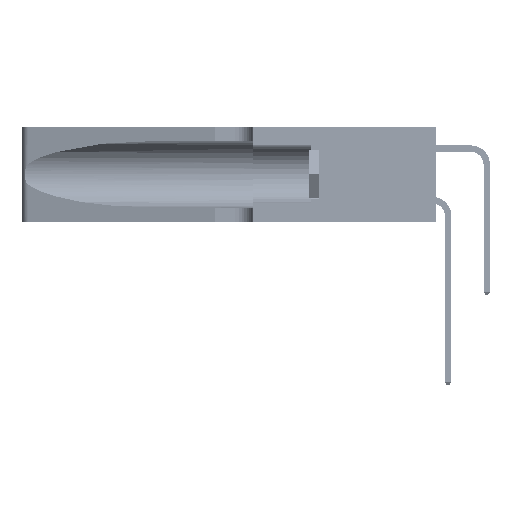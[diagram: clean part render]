
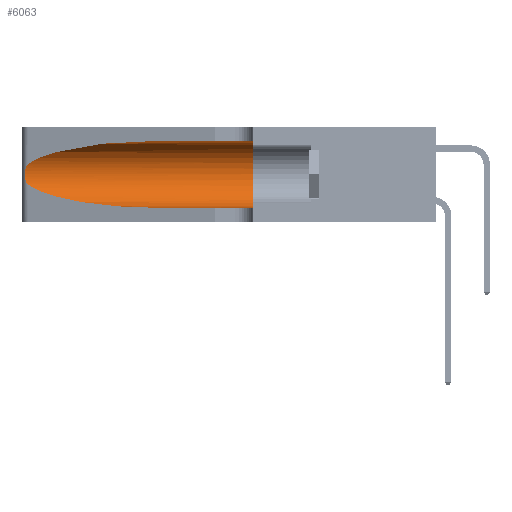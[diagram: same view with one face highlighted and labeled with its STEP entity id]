
A CAD part, left-side view. The second image highlights one B-rep face of the part: STEP entity #6063.
In plain terms, the highlighted cylindrical face has radius 3.308 mm (diameter 6.617 mm), a partial arc.
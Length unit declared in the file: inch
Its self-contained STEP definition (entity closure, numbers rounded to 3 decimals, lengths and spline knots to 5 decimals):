
#1471 = ORIENTED_EDGE ( 'NONE', *, *, #25149, .F. ) ;
#2690 = FACE_OUTER_BOUND ( 'NONE', #3818, .T. ) ;
#2762 = VERTEX_POINT ( 'NONE', #18186 ) ;
#2952 = CARTESIAN_POINT ( 'NONE',  ( 0.1305, 0.72297, 0.31525 ) ) ;
#3171 = CARTESIAN_POINT ( 'NONE',  ( 0.25787, 1.23484, 0.2124 ) ) ;
#3818 = EDGE_LOOP ( 'NONE', ( #35676, #42272, #21327, #41845, #1471, #45018 ) ) ;
#6063 = ADVANCED_FACE ( 'NONE', ( #2690 ), #40799, .F. ) ;
#6064 = AXIS2_PLACEMENT_3D ( 'NONE', #36379, #12071, #40425 ) ;
#6579 = EDGE_CURVE ( 'NONE', #7386, #30615, #22213, .T. ) ;
#7031 = DIRECTION ( 'NONE',  ( 0., 0., -1. ) ) ;
#7288 = CARTESIAN_POINT ( 'NONE',  ( 0.26018, 1.23835, 0.19895 ) ) ;
#7386 = VERTEX_POINT ( 'NONE', #46970 ) ;
#10471 =( BOUNDED_CURVE ( )  B_SPLINE_CURVE ( 3, ( #13249, #37545, #45640, #21408 ),
 .UNSPECIFIED., .F., .F. ) 
 B_SPLINE_CURVE_WITH_KNOTS ( ( 4, 4 ),
 ( 1.5708, 2.84003 ),
 .UNSPECIFIED. ) 
 CURVE ( )  GEOMETRIC_REPRESENTATION_ITEM ( )  RATIONAL_B_SPLINE_CURVE ( ( 1., 0.87, 0.87, 1. ) ) 
 REPRESENTATION_ITEM ( '' )  );
#11381 = CARTESIAN_POINT ( 'NONE',  ( 0.26075, 1.23896, 0.178 ) ) ;
#12071 = DIRECTION ( 'NONE',  ( 0., 1., 0. ) ) ;
#13249 = CARTESIAN_POINT ( 'NONE',  ( 0.1305, 0.72297, 0.31525 ) ) ;
#15060 = DIRECTION ( 'NONE',  ( 0., -1., 0. ) ) ;
#15468 = CARTESIAN_POINT ( 'NONE',  ( 0.25856, 1.23593, 0.16098 ) ) ;
#16273 = CARTESIAN_POINT ( 'NONE',  ( 0.25487, 1.22718, 0.22369 ) ) ;
#18186 = CARTESIAN_POINT ( 'NONE',  ( 0.1305, 0.35, 0.31525 ) ) ;
#18216 = CARTESIAN_POINT ( 'NONE',  ( 0.18966, 0.96281, 0.05475 ) ) ;
#18312 = B_SPLINE_CURVE_WITH_KNOTS ( 'NONE', 3,
 ( #43625, #39561, #27516, #3171, #31611, #7288, #35682, #11381, #39742, #15468, #43801, #19581, #47858, #23642 ),
 .UNSPECIFIED., .F., .F.,
 ( 4, 2, 2, 2, 2, 2, 4 ),
 ( 0., 0.00027, 0.00053, 0.00107, 0.0016, 0.00187, 0.00214 ),
 .UNSPECIFIED. ) ;
#19239 = DIRECTION ( 'NONE',  ( 0., -1., 0. ) ) ;
#19435 = EDGE_CURVE ( 'NONE', #36203, #7386, #18312, .T. ) ;
#19581 = CARTESIAN_POINT ( 'NONE',  ( 0.25639, 1.23186, 0.15144 ) ) ;
#21327 = ORIENTED_EDGE ( 'NONE', *, *, #6579, .T. ) ;
#21408 = CARTESIAN_POINT ( 'NONE',  ( 0.25487, 1.22718, 0.22369 ) ) ;
#22213 =( BOUNDED_CURVE ( )  B_SPLINE_CURVE ( 3, ( #22286, #46506, #18216, #26359 ),
 .UNSPECIFIED., .F., .F. ) 
 B_SPLINE_CURVE_WITH_KNOTS ( ( 4, 4 ),
 ( 3.44316, 4.71239 ),
 .UNSPECIFIED. ) 
 CURVE ( )  GEOMETRIC_REPRESENTATION_ITEM ( )  RATIONAL_B_SPLINE_CURVE ( ( 1., 0.87, 0.87, 1. ) ) 
 REPRESENTATION_ITEM ( '' )  );
#22286 = CARTESIAN_POINT ( 'NONE',  ( 0.25487, 1.22718, 0.14631 ) ) ;
#23642 = CARTESIAN_POINT ( 'NONE',  ( 0.25487, 1.22718, 0.14631 ) ) ;
#25149 = EDGE_CURVE ( 'NONE', #2762, #44845, #49588, .T. ) ;
#26359 = CARTESIAN_POINT ( 'NONE',  ( 0.1305, 0.72297, 0.05475 ) ) ;
#27516 = CARTESIAN_POINT ( 'NONE',  ( 0.25639, 1.23184, 0.21858 ) ) ;
#28360 = AXIS2_PLACEMENT_3D ( 'NONE', #47451, #31380, #7031 ) ;
#30157 = LINE ( 'NONE', #43477, #40908 ) ;
#30615 = VERTEX_POINT ( 'NONE', #38020 ) ;
#31380 = DIRECTION ( 'NONE',  ( 0., -1., 0. ) ) ;
#31528 = EDGE_CURVE ( 'NONE', #52019, #2762, #37275, .T. ) ;
#31611 = CARTESIAN_POINT ( 'NONE',  ( 0.25854, 1.2359, 0.20912 ) ) ;
#32174 = CARTESIAN_POINT ( 'NONE',  ( 0.1305, 0.35, 0.05475 ) ) ;
#32745 = EDGE_CURVE ( 'NONE', #30615, #44845, #30157, .T. ) ;
#34732 = VECTOR ( 'NONE', #15060, 39.37008 ) ;
#35676 = ORIENTED_EDGE ( 'NONE', *, *, #44424, .T. ) ;
#35682 = CARTESIAN_POINT ( 'NONE',  ( 0.26075, 1.23896, 0.19203 ) ) ;
#36203 = VERTEX_POINT ( 'NONE', #16273 ) ;
#36379 = CARTESIAN_POINT ( 'NONE',  ( 0.1305, 0.35, 0.185 ) ) ;
#37275 = LINE ( 'NONE', #47458, #34732 ) ;
#37545 = CARTESIAN_POINT ( 'NONE',  ( 0.18966, 0.96281, 0.31525 ) ) ;
#38020 = CARTESIAN_POINT ( 'NONE',  ( 0.1305, 0.72297, 0.05475 ) ) ;
#39561 = CARTESIAN_POINT ( 'NONE',  ( 0.25555, 1.22994, 0.2215 ) ) ;
#39742 = CARTESIAN_POINT ( 'NONE',  ( 0.26017, 1.23833, 0.17102 ) ) ;
#40425 = DIRECTION ( 'NONE',  ( 0., 0., 1. ) ) ;
#40799 = CYLINDRICAL_SURFACE ( 'NONE', #28360, 0.13025 ) ;
#40908 = VECTOR ( 'NONE', #19239, 39.37008 ) ;
#41845 = ORIENTED_EDGE ( 'NONE', *, *, #32745, .T. ) ;
#42272 = ORIENTED_EDGE ( 'NONE', *, *, #19435, .T. ) ;
#43477 = CARTESIAN_POINT ( 'NONE',  ( 0.1305, 1.61858, 0.05475 ) ) ;
#43625 = CARTESIAN_POINT ( 'NONE',  ( 0.25487, 1.22718, 0.22369 ) ) ;
#43801 = CARTESIAN_POINT ( 'NONE',  ( 0.25789, 1.23486, 0.15765 ) ) ;
#44424 = EDGE_CURVE ( 'NONE', #52019, #36203, #10471, .T. ) ;
#44845 = VERTEX_POINT ( 'NONE', #32174 ) ;
#45018 = ORIENTED_EDGE ( 'NONE', *, *, #31528, .F. ) ;
#45640 = CARTESIAN_POINT ( 'NONE',  ( 0.2373, 1.15595, 0.28018 ) ) ;
#46506 = CARTESIAN_POINT ( 'NONE',  ( 0.2373, 1.15595, 0.08982 ) ) ;
#46970 = CARTESIAN_POINT ( 'NONE',  ( 0.25487, 1.22718, 0.14631 ) ) ;
#47451 = CARTESIAN_POINT ( 'NONE',  ( 0.1305, 1.61858, 0.185 ) ) ;
#47458 = CARTESIAN_POINT ( 'NONE',  ( 0.1305, 1.61858, 0.31525 ) ) ;
#47858 = CARTESIAN_POINT ( 'NONE',  ( 0.25555, 1.22993, 0.14849 ) ) ;
#49588 = CIRCLE ( 'NONE', #6064, 0.13025 ) ;
#52019 = VERTEX_POINT ( 'NONE', #2952 ) ;
